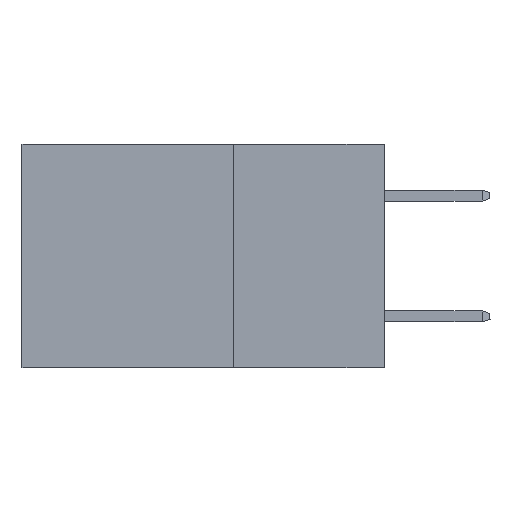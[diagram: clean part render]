
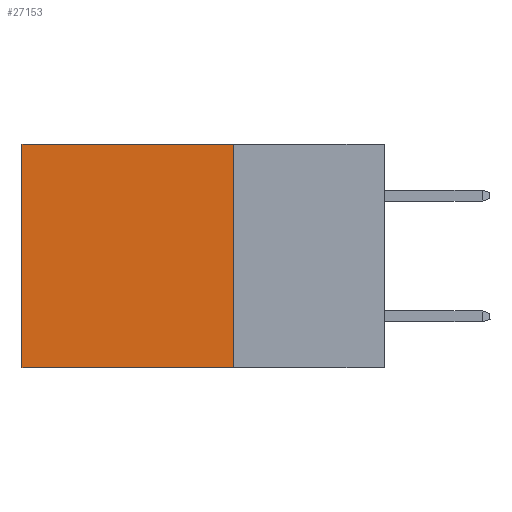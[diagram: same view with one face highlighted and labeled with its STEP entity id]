
A CAD part, left-side view. The second image highlights one B-rep face of the part: STEP entity #27153.
In plain terms, the highlighted planar face has unit normal (-1, 0, 0).
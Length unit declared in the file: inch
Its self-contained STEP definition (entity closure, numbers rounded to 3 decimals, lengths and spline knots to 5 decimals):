
#1861 = VECTOR ( 'NONE', #11580, 39.37008 ) ;
#2253 = EDGE_LOOP ( 'NONE', ( #6531, #4801, #17434, #19369 ) ) ;
#2706 = VERTEX_POINT ( 'NONE', #18149 ) ;
#2726 = PLANE ( 'NONE',  #13656 ) ;
#3033 = VERTEX_POINT ( 'NONE', #4080 ) ;
#3228 = LINE ( 'NONE', #9419, #1861 ) ;
#4080 = CARTESIAN_POINT ( 'NONE',  ( 0.2615, 0.6, 0. ) ) ;
#4504 = EDGE_CURVE ( 'NONE', #17630, #19929, #12125, .T. ) ;
#4801 = ORIENTED_EDGE ( 'NONE', *, *, #4504, .F. ) ;
#5745 = DIRECTION ( 'NONE',  ( 0., 1., 0. ) ) ;
#5810 = EDGE_CURVE ( 'NONE', #3033, #19929, #3228, .T. ) ;
#6531 = ORIENTED_EDGE ( 'NONE', *, *, #5810, .T. ) ;
#7101 = DIRECTION ( 'NONE',  ( 0., 0., -1. ) ) ;
#7918 = CARTESIAN_POINT ( 'NONE',  ( 0.2615, 0.25, 0. ) ) ;
#9419 = CARTESIAN_POINT ( 'NONE',  ( 0.2615, 0.6, -0.37 ) ) ;
#11241 = LINE ( 'NONE', #14890, #26762 ) ;
#11580 = DIRECTION ( 'NONE',  ( 0., 0., -1. ) ) ;
#12125 = LINE ( 'NONE', #22621, #16465 ) ;
#13656 = AXIS2_PLACEMENT_3D ( 'NONE', #17836, #19989, #7101 ) ;
#14890 = CARTESIAN_POINT ( 'NONE',  ( 0.2615, 0.25, -0.37 ) ) ;
#16465 = VECTOR ( 'NONE', #24698, 39.37008 ) ;
#17051 = DIRECTION ( 'NONE',  ( 0., 0., -1. ) ) ;
#17434 = ORIENTED_EDGE ( 'NONE', *, *, #27580, .F. ) ;
#17630 = VERTEX_POINT ( 'NONE', #23109 ) ;
#17836 = CARTESIAN_POINT ( 'NONE',  ( 0.2615, 0.25, -0.37 ) ) ;
#18149 = CARTESIAN_POINT ( 'NONE',  ( 0.2615, 0.25, 0. ) ) ;
#19369 = ORIENTED_EDGE ( 'NONE', *, *, #22332, .T. ) ;
#19929 = VERTEX_POINT ( 'NONE', #23503 ) ;
#19989 = DIRECTION ( 'NONE',  ( 1., 0., 0. ) ) ;
#22332 = EDGE_CURVE ( 'NONE', #2706, #3033, #26629, .T. ) ;
#22590 = FACE_OUTER_BOUND ( 'NONE', #2253, .T. ) ;
#22621 = CARTESIAN_POINT ( 'NONE',  ( 0.2615, 0.25, -0.37 ) ) ;
#23109 = CARTESIAN_POINT ( 'NONE',  ( 0.2615, 0.25, -0.37 ) ) ;
#23503 = CARTESIAN_POINT ( 'NONE',  ( 0.2615, 0.6, -0.37 ) ) ;
#24698 = DIRECTION ( 'NONE',  ( 0., 1., 0. ) ) ;
#25987 = VECTOR ( 'NONE', #5745, 39.37008 ) ;
#26629 = LINE ( 'NONE', #7918, #25987 ) ;
#26762 = VECTOR ( 'NONE', #17051, 39.37008 ) ;
#27153 = ADVANCED_FACE ( 'NONE', ( #22590 ), #2726, .F. ) ;
#27580 = EDGE_CURVE ( 'NONE', #2706, #17630, #11241, .T. ) ;
